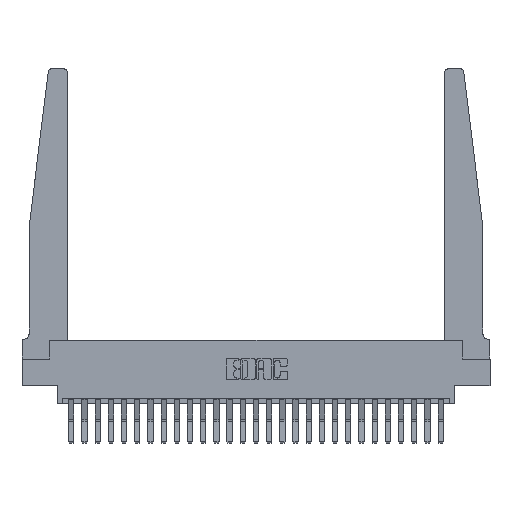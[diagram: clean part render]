
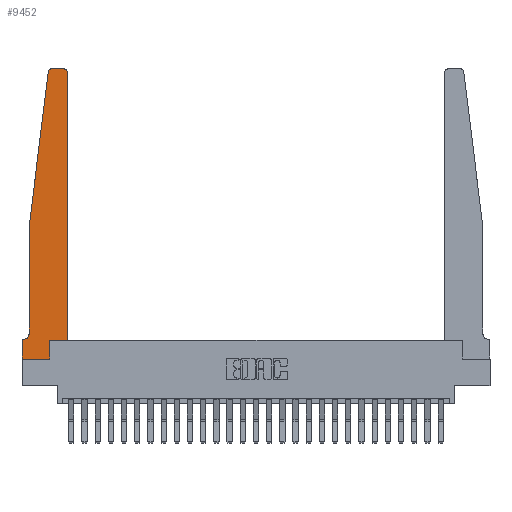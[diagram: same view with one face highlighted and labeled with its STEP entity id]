
A CAD part, top view. The second image highlights one B-rep face of the part: STEP entity #9452.
In plain terms, the highlighted planar face has unit normal (0, 0, 1).
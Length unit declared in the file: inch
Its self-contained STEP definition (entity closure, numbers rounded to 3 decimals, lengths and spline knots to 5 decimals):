
#251 = CARTESIAN_POINT ( 'NONE',  ( 0.27653, 2.72, 0.37 ) ) ;
#318 = ORIENTED_EDGE ( 'NONE', *, *, #20460, .T. ) ;
#388 = EDGE_CURVE ( 'NONE', #13076, #4066, #12016, .T. ) ;
#435 = VERTEX_POINT ( 'NONE', #10681 ) ;
#446 = DIRECTION ( 'NONE',  ( 1., 0., 0. ) ) ;
#872 = DIRECTION ( 'NONE',  ( 0., 1., 0. ) ) ;
#996 = CARTESIAN_POINT ( 'NONE',  ( 0.065, 1.25, 0.37 ) ) ;
#1075 = EDGE_CURVE ( 'NONE', #4066, #20961, #24246, .T. ) ;
#1227 = EDGE_CURVE ( 'NONE', #5909, #13076, #5965, .T. ) ;
#1235 = ORIENTED_EDGE ( 'NONE', *, *, #1718, .T. ) ;
#1718 = EDGE_CURVE ( 'NONE', #20961, #8485, #22104, .T. ) ;
#1955 = VERTEX_POINT ( 'NONE', #24720 ) ;
#2235 = DIRECTION ( 'NONE',  ( 1., 0., 0. ) ) ;
#2473 = ORIENTED_EDGE ( 'NONE', *, *, #13269, .T. ) ;
#3052 = AXIS2_PLACEMENT_3D ( 'NONE', #251, #14322, #2235 ) ;
#3056 = EDGE_CURVE ( 'NONE', #435, #1955, #21413, .T. ) ;
#3764 = LINE ( 'NONE', #18404, #19140 ) ;
#3953 = CARTESIAN_POINT ( 'NONE',  ( 0.425, 2.72, 0.37 ) ) ;
#4066 = VERTEX_POINT ( 'NONE', #8910 ) ;
#4133 = CARTESIAN_POINT ( 'NONE',  ( 0.065, 1.25, 0.37 ) ) ;
#4218 = CARTESIAN_POINT ( 'NONE',  ( 0.425, 0.18, 0.37 ) ) ;
#4399 = DIRECTION ( 'NONE',  ( 0., 0., 1. ) ) ;
#4737 = EDGE_CURVE ( 'NONE', #21432, #7384, #21631, .T. ) ;
#4993 = ORIENTED_EDGE ( 'NONE', *, *, #3056, .T. ) ;
#4994 = CARTESIAN_POINT ( 'NONE',  ( 0.425, 0.18, 0.37 ) ) ;
#5084 = CARTESIAN_POINT ( 'NONE',  ( 0.015, 0.2375, 0.37 ) ) ;
#5321 = VECTOR ( 'NONE', #872, 39.37008 ) ;
#5340 = ORIENTED_EDGE ( 'NONE', *, *, #388, .T. ) ;
#5645 = ORIENTED_EDGE ( 'NONE', *, *, #4737, .T. ) ;
#5909 = VERTEX_POINT ( 'NONE', #4994 ) ;
#5965 = LINE ( 'NONE', #10984, #5321 ) ;
#7143 = DIRECTION ( 'NONE',  ( -1., 0., 0. ) ) ;
#7384 = VERTEX_POINT ( 'NONE', #18269 ) ;
#7551 = CARTESIAN_POINT ( 'NONE',  ( 0.2605, 0., 0.37 ) ) ;
#8270 = EDGE_LOOP ( 'NONE', ( #16023, #1235, #12010, #2473, #4993, #318, #5645, #17588, #12951, #18816, #10166, #5340 ) ) ;
#8411 = VERTEX_POINT ( 'NONE', #7551 ) ;
#8485 = VERTEX_POINT ( 'NONE', #23626 ) ;
#8541 = VECTOR ( 'NONE', #16517, 39.37008 ) ;
#8910 = CARTESIAN_POINT ( 'NONE',  ( 0.395, 2.75, 0.37 ) ) ;
#9167 = DIRECTION ( 'NONE',  ( 0., -1., 0. ) ) ;
#9452 = ADVANCED_FACE ( 'NONE', ( #24321 ), #24251, .T. ) ;
#9588 = CARTESIAN_POINT ( 'NONE',  ( 0., 0., 0.37 ) ) ;
#9992 = CARTESIAN_POINT ( 'NONE',  ( 0.27653, 2.75, 0.37 ) ) ;
#10166 = ORIENTED_EDGE ( 'NONE', *, *, #1227, .T. ) ;
#10331 = DIRECTION ( 'NONE',  ( -0.122, -0.992, 0. ) ) ;
#10681 = CARTESIAN_POINT ( 'NONE',  ( 0.065, 0.2375, 0.37 ) ) ;
#10765 = EDGE_CURVE ( 'NONE', #24568, #5909, #21550, .T. ) ;
#10984 = CARTESIAN_POINT ( 'NONE',  ( 0.425, 0.18, 0.37 ) ) ;
#11112 = EDGE_CURVE ( 'NONE', #8485, #21092, #20007, .T. ) ;
#11117 = VECTOR ( 'NONE', #14301, 39.37008 ) ;
#11805 = DIRECTION ( 'NONE',  ( 1., 0., 0. ) ) ;
#12010 = ORIENTED_EDGE ( 'NONE', *, *, #11112, .T. ) ;
#12016 = CIRCLE ( 'NONE', #14535, 0.03 ) ;
#12554 = DIRECTION ( 'NONE',  ( 0., 0., 1. ) ) ;
#12951 = ORIENTED_EDGE ( 'NONE', *, *, #17389, .T. ) ;
#13076 = VERTEX_POINT ( 'NONE', #3953 ) ;
#13269 = EDGE_CURVE ( 'NONE', #21092, #435, #24716, .T. ) ;
#14301 = DIRECTION ( 'NONE',  ( 1., 0., 0. ) ) ;
#14322 = DIRECTION ( 'NONE',  ( 0., 0., 1. ) ) ;
#14535 = AXIS2_PLACEMENT_3D ( 'NONE', #16470, #4399, #18443 ) ;
#15574 = DIRECTION ( 'NONE',  ( 0., -1., 0. ) ) ;
#15872 = CARTESIAN_POINT ( 'NONE',  ( 0.2605, 0.18, 0.37 ) ) ;
#16023 = ORIENTED_EDGE ( 'NONE', *, *, #1075, .T. ) ;
#16432 = DIRECTION ( 'NONE',  ( -1., 0., 0. ) ) ;
#16470 = CARTESIAN_POINT ( 'NONE',  ( 0.395, 2.72, 0.37 ) ) ;
#16481 = VECTOR ( 'NONE', #11805, 39.37008 ) ;
#16486 = CARTESIAN_POINT ( 'NONE',  ( 0.065, 1.25, 0.37 ) ) ;
#16517 = DIRECTION ( 'NONE',  ( -1., 0., 0. ) ) ;
#17110 = LINE ( 'NONE', #21582, #16481 ) ;
#17389 = EDGE_CURVE ( 'NONE', #8411, #24568, #23353, .T. ) ;
#17588 = ORIENTED_EDGE ( 'NONE', *, *, #25022, .T. ) ;
#17768 = CARTESIAN_POINT ( 'NONE',  ( 0., 0.1875, 0.37 ) ) ;
#17849 = DIRECTION ( 'NONE',  ( 0., 1., 0. ) ) ;
#18186 = VECTOR ( 'NONE', #17849, 39.37008 ) ;
#18269 = CARTESIAN_POINT ( 'NONE',  ( 0., 0., 0.37 ) ) ;
#18296 = CARTESIAN_POINT ( 'NONE',  ( 0.2605, 0.18, 0.37 ) ) ;
#18404 = CARTESIAN_POINT ( 'NONE',  ( 0.065, 0.1875, 0.37 ) ) ;
#18443 = DIRECTION ( 'NONE',  ( 1., 0., 0. ) ) ;
#18816 = ORIENTED_EDGE ( 'NONE', *, *, #10765, .T. ) ;
#19030 = AXIS2_PLACEMENT_3D ( 'NONE', #20360, #12554, #446 ) ;
#19105 = DIRECTION ( 'NONE',  ( 0., 0., -1. ) ) ;
#19140 = VECTOR ( 'NONE', #16432, 39.37008 ) ;
#19414 = VECTOR ( 'NONE', #10331, 39.37008 ) ;
#19566 = VECTOR ( 'NONE', #9167, 39.37008 ) ;
#20007 = LINE ( 'NONE', #4133, #19414 ) ;
#20360 = CARTESIAN_POINT ( 'NONE',  ( 0., 0.1875, 0.37 ) ) ;
#20412 = VECTOR ( 'NONE', #15574, 39.37008 ) ;
#20460 = EDGE_CURVE ( 'NONE', #1955, #21432, #3764, .T. ) ;
#20961 = VERTEX_POINT ( 'NONE', #9992 ) ;
#21092 = VERTEX_POINT ( 'NONE', #16486 ) ;
#21413 = CIRCLE ( 'NONE', #21620, 0.05 ) ;
#21432 = VERTEX_POINT ( 'NONE', #17768 ) ;
#21550 = LINE ( 'NONE', #4218, #11117 ) ;
#21582 = CARTESIAN_POINT ( 'NONE',  ( 0., 0., 0.37 ) ) ;
#21620 = AXIS2_PLACEMENT_3D ( 'NONE', #5084, #19105, #7143 ) ;
#21631 = LINE ( 'NONE', #9588, #20412 ) ;
#22104 = CIRCLE ( 'NONE', #3052, 0.03 ) ;
#23353 = LINE ( 'NONE', #15872, #18186 ) ;
#23626 = CARTESIAN_POINT ( 'NONE',  ( 0.24675, 2.72367, 0.37 ) ) ;
#24244 = CARTESIAN_POINT ( 'NONE',  ( 0.25, 2.75, 0.37 ) ) ;
#24246 = LINE ( 'NONE', #24244, #8541 ) ;
#24251 = PLANE ( 'NONE',  #19030 ) ;
#24321 = FACE_OUTER_BOUND ( 'NONE', #8270, .T. ) ;
#24568 = VERTEX_POINT ( 'NONE', #18296 ) ;
#24716 = LINE ( 'NONE', #996, #19566 ) ;
#24720 = CARTESIAN_POINT ( 'NONE',  ( 0.015, 0.1875, 0.37 ) ) ;
#25022 = EDGE_CURVE ( 'NONE', #7384, #8411, #17110, .T. ) ;
